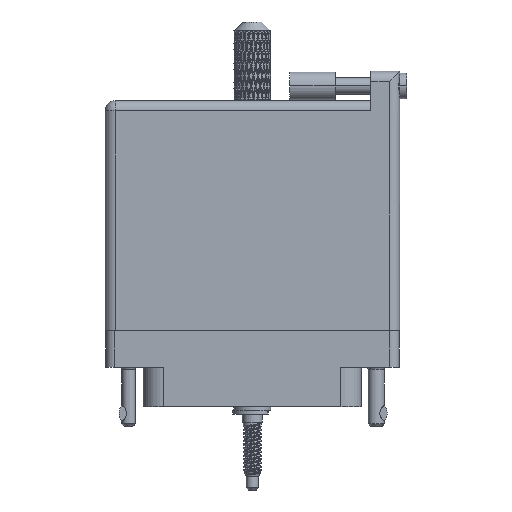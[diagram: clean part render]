
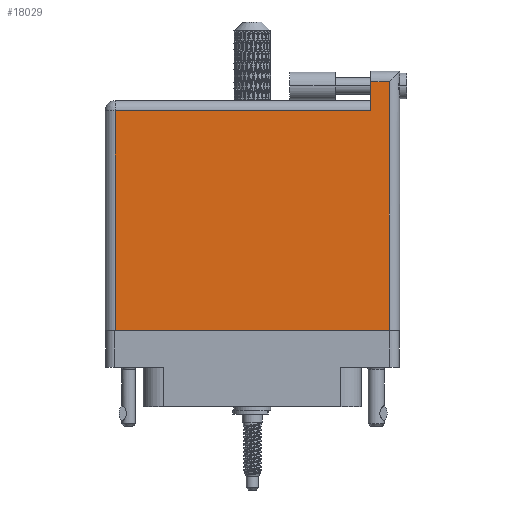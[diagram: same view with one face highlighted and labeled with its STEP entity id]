
A CAD part, front view. The second image highlights one B-rep face of the part: STEP entity #18029.
In plain terms, the highlighted face is planar.
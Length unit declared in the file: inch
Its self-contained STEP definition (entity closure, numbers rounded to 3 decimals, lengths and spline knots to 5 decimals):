
#79 = DIRECTION ( 'NONE',  ( 0., 0., -1. ) ) ;
#1511 = CARTESIAN_POINT ( 'NONE',  ( -0.934, -0.1, 0.4495 ) ) ;
#2595 = CARTESIAN_POINT ( 'NONE',  ( -0.934, -0.1, 0.4495 ) ) ;
#3088 = CARTESIAN_POINT ( 'NONE',  ( -0.934, 1.396, 0.4495 ) ) ;
#6474 = VERTEX_POINT ( 'NONE', #84330 ) ;
#7131 = CARTESIAN_POINT ( 'NONE',  ( 0.934, 1.666, 0.4495 ) ) ;
#7352 = FACE_OUTER_BOUND ( 'NONE', #92439, .T. ) ;
#9372 = DIRECTION ( 'NONE',  ( -1., 0., 0. ) ) ;
#11688 = LINE ( 'NONE', #38448, #107312 ) ;
#18029 = ADVANCED_FACE ( 'NONE', ( #7352 ), #51175, .F. ) ;
#18989 = EDGE_CURVE ( 'NONE', #100409, #56136, #19684, .T. ) ;
#19560 = EDGE_CURVE ( 'NONE', #79517, #113972, #61078, .T. ) ;
#19684 = LINE ( 'NONE', #1511, #68078 ) ;
#22583 = ORIENTED_EDGE ( 'NONE', *, *, #97930, .T. ) ;
#25038 = ORIENTED_EDGE ( 'NONE', *, *, #19560, .T. ) ;
#27034 = AXIS2_PLACEMENT_3D ( 'NONE', #35333, #79, #9372 ) ;
#32767 = CARTESIAN_POINT ( 'NONE',  ( -1.004, -0.1, 0.4495 ) ) ;
#33108 = VECTOR ( 'NONE', #53003, 39.37008 ) ;
#34628 = DIRECTION ( 'NONE',  ( 0., 1., 0. ) ) ;
#35333 = CARTESIAN_POINT ( 'NONE',  ( -1.004, 1.466, 0.4495 ) ) ;
#36867 = ORIENTED_EDGE ( 'NONE', *, *, #93878, .T. ) ;
#37695 = DIRECTION ( 'NONE',  ( -1., 0., 0. ) ) ;
#38448 = CARTESIAN_POINT ( 'NONE',  ( -1.004, 1.596, 0.4495 ) ) ;
#39498 = DIRECTION ( 'NONE',  ( 0., -1., 0. ) ) ;
#42815 = CARTESIAN_POINT ( 'NONE',  ( 0.934, -0.1, 0.4495 ) ) ;
#45009 = LINE ( 'NONE', #32767, #95033 ) ;
#45997 = VECTOR ( 'NONE', #39498, 39.37008 ) ;
#51175 = PLANE ( 'NONE',  #27034 ) ;
#51421 = CARTESIAN_POINT ( 'NONE',  ( 0.934, 1.596, 0.4495 ) ) ;
#52396 = LINE ( 'NONE', #114656, #33108 ) ;
#53003 = DIRECTION ( 'NONE',  ( -1., 0., 0. ) ) ;
#53326 = EDGE_CURVE ( 'NONE', #56136, #79517, #45009, .T. ) ;
#56136 = VERTEX_POINT ( 'NONE', #2595 ) ;
#58303 = ORIENTED_EDGE ( 'NONE', *, *, #18989, .T. ) ;
#61078 = LINE ( 'NONE', #7131, #101399 ) ;
#63257 = ORIENTED_EDGE ( 'NONE', *, *, #77673, .T. ) ;
#68051 = LINE ( 'NONE', #92659, #45997 ) ;
#68078 = VECTOR ( 'NONE', #81300, 39.37008 ) ;
#75869 = VERTEX_POINT ( 'NONE', #110824 ) ;
#77673 = EDGE_CURVE ( 'NONE', #75869, #6474, #68051, .T. ) ;
#79099 = ORIENTED_EDGE ( 'NONE', *, *, #53326, .T. ) ;
#79517 = VERTEX_POINT ( 'NONE', #42815 ) ;
#81300 = DIRECTION ( 'NONE',  ( 0., -1., 0. ) ) ;
#84330 = CARTESIAN_POINT ( 'NONE',  ( 0.807, 1.396, 0.4495 ) ) ;
#92439 = EDGE_LOOP ( 'NONE', ( #79099, #25038, #22583, #63257, #36867, #58303 ) ) ;
#92659 = CARTESIAN_POINT ( 'NONE',  ( 0.807, 1.666, 0.4495 ) ) ;
#93878 = EDGE_CURVE ( 'NONE', #6474, #100409, #52396, .T. ) ;
#95033 = VECTOR ( 'NONE', #112161, 39.37008 ) ;
#97930 = EDGE_CURVE ( 'NONE', #113972, #75869, #11688, .T. ) ;
#100409 = VERTEX_POINT ( 'NONE', #3088 ) ;
#101399 = VECTOR ( 'NONE', #34628, 39.37008 ) ;
#107312 = VECTOR ( 'NONE', #37695, 39.37008 ) ;
#110824 = CARTESIAN_POINT ( 'NONE',  ( 0.807, 1.596, 0.4495 ) ) ;
#112161 = DIRECTION ( 'NONE',  ( 1., 0., 0. ) ) ;
#113972 = VERTEX_POINT ( 'NONE', #51421 ) ;
#114656 = CARTESIAN_POINT ( 'NONE',  ( -1.004, 1.396, 0.4495 ) ) ;
